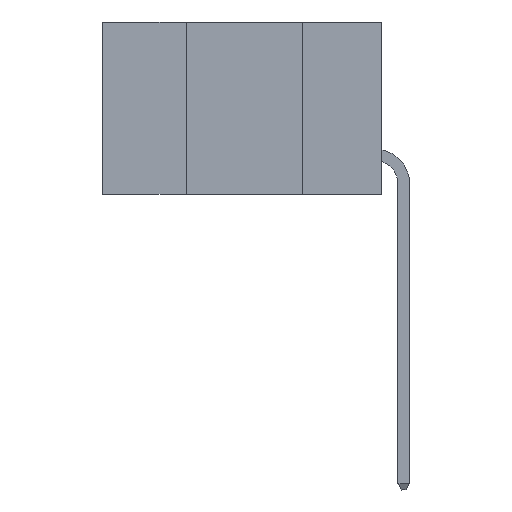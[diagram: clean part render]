
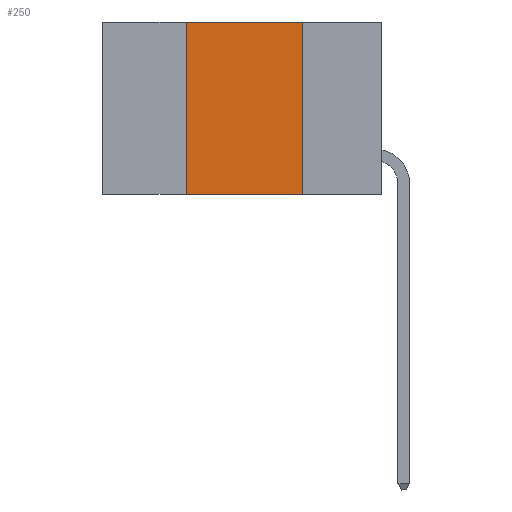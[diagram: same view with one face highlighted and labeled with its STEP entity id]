
A CAD part, left-side view. The second image highlights one B-rep face of the part: STEP entity #250.
In plain terms, the highlighted planar face has unit normal (-1, 0, 0).
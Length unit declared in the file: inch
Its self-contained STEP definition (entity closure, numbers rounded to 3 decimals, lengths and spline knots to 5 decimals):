
#10 = LINE ( 'NONE', #9022, #6470 ) ;
#250 = ADVANCED_FACE ( 'NONE', ( #8708 ), #5515, .F. ) ;
#391 = EDGE_CURVE ( 'NONE', #10195, #7521, #9033, .T. ) ;
#414 = ORIENTED_EDGE ( 'NONE', *, *, #5581, .F. ) ;
#423 = LINE ( 'NONE', #8687, #1010 ) ;
#605 = CARTESIAN_POINT ( 'NONE',  ( 0., 0.17, 0. ) ) ;
#1010 = VECTOR ( 'NONE', #3383, 39.37008 ) ;
#1530 = CARTESIAN_POINT ( 'NONE',  ( 0., 0.17, 0. ) ) ;
#1761 = AXIS2_PLACEMENT_3D ( 'NONE', #5447, #5498, #5489 ) ;
#1867 = LINE ( 'NONE', #605, #7709 ) ;
#1959 = VERTEX_POINT ( 'NONE', #1530 ) ;
#2487 = VERTEX_POINT ( 'NONE', #9100 ) ;
#3278 = DIRECTION ( 'NONE',  ( 0., 0., -1. ) ) ;
#3383 = DIRECTION ( 'NONE',  ( 0., -1., 0. ) ) ;
#3387 = CARTESIAN_POINT ( 'NONE',  ( 0., 0.42, 0. ) ) ;
#3495 = VECTOR ( 'NONE', #3589, 39.37008 ) ;
#3589 = DIRECTION ( 'NONE',  ( 0., 0., 1. ) ) ;
#4103 = EDGE_CURVE ( 'NONE', #10195, #2487, #10, .T. ) ;
#4670 = ORIENTED_EDGE ( 'NONE', *, *, #4103, .T. ) ;
#4731 = ORIENTED_EDGE ( 'NONE', *, *, #5501, .F. ) ;
#4739 = ORIENTED_EDGE ( 'NONE', *, *, #391, .F. ) ;
#5447 = CARTESIAN_POINT ( 'NONE',  ( 0., 0.6, 0. ) ) ;
#5489 = DIRECTION ( 'NONE',  ( 0., 0., -1. ) ) ;
#5498 = DIRECTION ( 'NONE',  ( 1., 0., 0. ) ) ;
#5501 = EDGE_CURVE ( 'NONE', #1959, #2487, #1867, .T. ) ;
#5515 = PLANE ( 'NONE',  #1761 ) ;
#5581 = EDGE_CURVE ( 'NONE', #7521, #1959, #423, .T. ) ;
#6299 = EDGE_LOOP ( 'NONE', ( #4731, #414, #4739, #4670 ) ) ;
#6470 = VECTOR ( 'NONE', #9737, 39.37008 ) ;
#6635 = CARTESIAN_POINT ( 'NONE',  ( 0., 0.42, 0. ) ) ;
#7521 = VERTEX_POINT ( 'NONE', #6635 ) ;
#7709 = VECTOR ( 'NONE', #3278, 39.37008 ) ;
#8687 = CARTESIAN_POINT ( 'NONE',  ( 0., 0.6, 0. ) ) ;
#8708 = FACE_OUTER_BOUND ( 'NONE', #6299, .T. ) ;
#9022 = CARTESIAN_POINT ( 'NONE',  ( 0., 0.6, -0.37 ) ) ;
#9033 = LINE ( 'NONE', #3387, #3495 ) ;
#9100 = CARTESIAN_POINT ( 'NONE',  ( 0., 0.17, -0.37 ) ) ;
#9737 = DIRECTION ( 'NONE',  ( 0., -1., 0. ) ) ;
#9919 = CARTESIAN_POINT ( 'NONE',  ( 0., 0.42, -0.37 ) ) ;
#10195 = VERTEX_POINT ( 'NONE', #9919 ) ;
